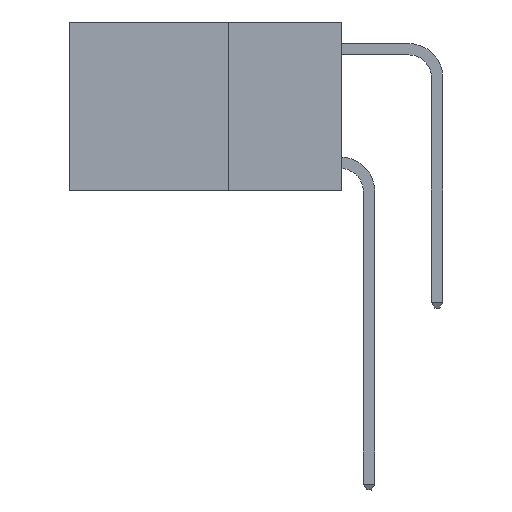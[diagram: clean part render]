
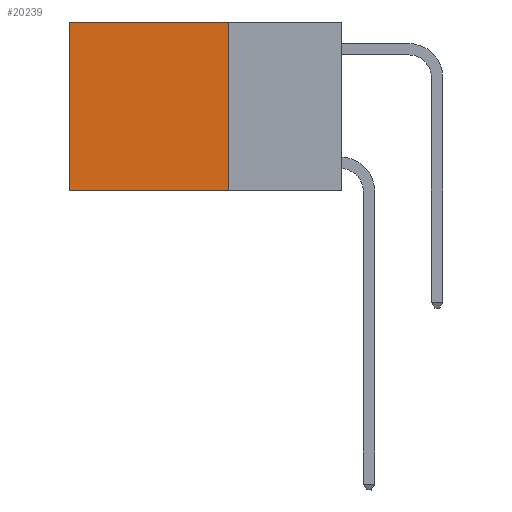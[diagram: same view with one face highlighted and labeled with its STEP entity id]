
A CAD part, left-side view. The second image highlights one B-rep face of the part: STEP entity #20239.
In plain terms, the highlighted planar face has unit normal (-1, 0, 0).
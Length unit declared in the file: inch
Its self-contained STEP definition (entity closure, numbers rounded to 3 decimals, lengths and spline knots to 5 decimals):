
#1853 = PLANE ( 'NONE',  #5516 ) ;
#2670 = DIRECTION ( 'NONE',  ( 0., 1., 0. ) ) ;
#2731 = LINE ( 'NONE', #10461, #23141 ) ;
#2824 = DIRECTION ( 'NONE',  ( 0., 1., 0. ) ) ;
#3562 = CARTESIAN_POINT ( 'NONE',  ( 0.2625, 0.6, -0.37 ) ) ;
#3707 = VERTEX_POINT ( 'NONE', #7286 ) ;
#5500 = ORIENTED_EDGE ( 'NONE', *, *, #24210, .F. ) ;
#5516 = AXIS2_PLACEMENT_3D ( 'NONE', #9579, #23101, #17300 ) ;
#6389 = VERTEX_POINT ( 'NONE', #10111 ) ;
#6805 = VERTEX_POINT ( 'NONE', #17417 ) ;
#7286 = CARTESIAN_POINT ( 'NONE',  ( 0.2625, 0.25, -0.37 ) ) ;
#9579 = CARTESIAN_POINT ( 'NONE',  ( 0.2625, 0.25, 0. ) ) ;
#10111 = CARTESIAN_POINT ( 'NONE',  ( 0.2625, 0.25, 0. ) ) ;
#10298 = EDGE_CURVE ( 'NONE', #6805, #12682, #2731, .T. ) ;
#10461 = CARTESIAN_POINT ( 'NONE',  ( 0.2625, 0.6, 0. ) ) ;
#10578 = DIRECTION ( 'NONE',  ( 0., 0., -1. ) ) ;
#10860 = VECTOR ( 'NONE', #15781, 39.37008 ) ;
#12293 = LINE ( 'NONE', #20498, #15362 ) ;
#12682 = VERTEX_POINT ( 'NONE', #3562 ) ;
#13654 = ORIENTED_EDGE ( 'NONE', *, *, #19469, .F. ) ;
#13749 = FACE_OUTER_BOUND ( 'NONE', #17822, .T. ) ;
#15362 = VECTOR ( 'NONE', #2670, 39.37008 ) ;
#15781 = DIRECTION ( 'NONE',  ( 0., 0., -1. ) ) ;
#16600 = CARTESIAN_POINT ( 'NONE',  ( 0.2625, 0.25, 0. ) ) ;
#17300 = DIRECTION ( 'NONE',  ( 0., 0., -1. ) ) ;
#17417 = CARTESIAN_POINT ( 'NONE',  ( 0.2625, 0.6, 0. ) ) ;
#17822 = EDGE_LOOP ( 'NONE', ( #19866, #13654, #5500, #20600 ) ) ;
#18518 = LINE ( 'NONE', #16600, #21724 ) ;
#19442 = LINE ( 'NONE', #19825, #10860 ) ;
#19469 = EDGE_CURVE ( 'NONE', #3707, #12682, #12293, .T. ) ;
#19825 = CARTESIAN_POINT ( 'NONE',  ( 0.2625, 0.25, 0. ) ) ;
#19866 = ORIENTED_EDGE ( 'NONE', *, *, #10298, .T. ) ;
#20239 = ADVANCED_FACE ( 'NONE', ( #13749 ), #1853, .F. ) ;
#20498 = CARTESIAN_POINT ( 'NONE',  ( 0.2625, 0.25, -0.37 ) ) ;
#20600 = ORIENTED_EDGE ( 'NONE', *, *, #21731, .T. ) ;
#21724 = VECTOR ( 'NONE', #2824, 39.37008 ) ;
#21731 = EDGE_CURVE ( 'NONE', #6389, #6805, #18518, .T. ) ;
#23101 = DIRECTION ( 'NONE',  ( 1., 0., 0. ) ) ;
#23141 = VECTOR ( 'NONE', #10578, 39.37008 ) ;
#24210 = EDGE_CURVE ( 'NONE', #6389, #3707, #19442, .T. ) ;
